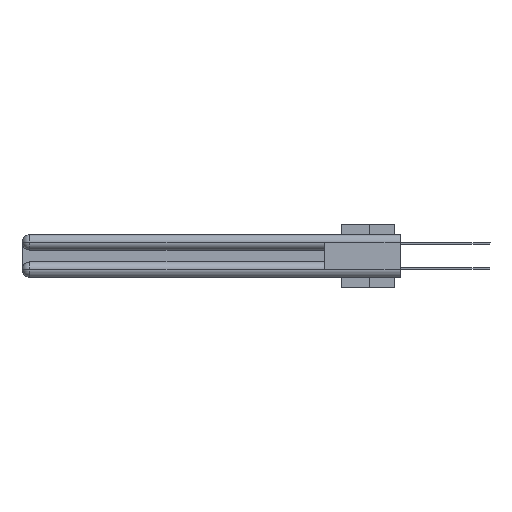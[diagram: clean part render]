
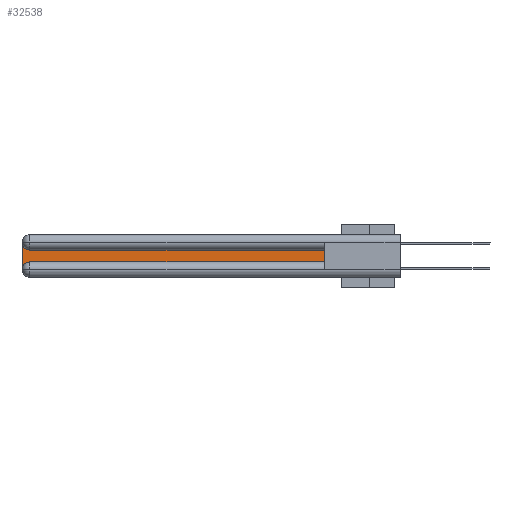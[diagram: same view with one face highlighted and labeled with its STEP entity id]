
A CAD part, left-side view. The second image highlights one B-rep face of the part: STEP entity #32538.
In plain terms, the highlighted planar face has unit normal (-1, 0, 0).
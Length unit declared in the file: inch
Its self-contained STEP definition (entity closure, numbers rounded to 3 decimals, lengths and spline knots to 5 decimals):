
#43 = AXIS2_PLACEMENT_3D ( 'NONE', #26752, #15834, #15995 ) ;
#588 = VECTOR ( 'NONE', #11236, 39.37008 ) ;
#1781 = DIRECTION ( 'NONE',  ( 1., 0., 0. ) ) ;
#1856 = VECTOR ( 'NONE', #23409, 39.37008 ) ;
#2509 = CARTESIAN_POINT ( 'NONE',  ( 0.075, 3., -0.2175 ) ) ;
#3250 = EDGE_CURVE ( 'NONE', #16935, #15985, #17031, .T. ) ;
#3287 = CIRCLE ( 'NONE', #22973, 0.06 ) ;
#3615 = ORIENTED_EDGE ( 'NONE', *, *, #17392, .T. ) ;
#4435 = CARTESIAN_POINT ( 'NONE',  ( 0.075, 3., -0.2775 ) ) ;
#5384 = FACE_OUTER_BOUND ( 'NONE', #6794, .T. ) ;
#5466 = VERTEX_POINT ( 'NONE', #32151 ) ;
#6429 = CARTESIAN_POINT ( 'NONE',  ( 0.075, 2.94, -0.0625 ) ) ;
#6794 = EDGE_LOOP ( 'NONE', ( #24310, #8093, #25225, #15275, #3615, #29367 ) ) ;
#6808 = VERTEX_POINT ( 'NONE', #4435 ) ;
#8093 = ORIENTED_EDGE ( 'NONE', *, *, #3250, .T. ) ;
#8192 = EDGE_CURVE ( 'NONE', #15985, #6808, #25975, .T. ) ;
#8545 = LINE ( 'NONE', #20891, #24804 ) ;
#8816 = LINE ( 'NONE', #26793, #588 ) ;
#10789 = DIRECTION ( 'NONE',  ( 0., -1., 0. ) ) ;
#11079 = CARTESIAN_POINT ( 'NONE',  ( 0.075, 0.6, -0.2175 ) ) ;
#11236 = DIRECTION ( 'NONE',  ( 0., 1., 0. ) ) ;
#12246 = DIRECTION ( 'NONE',  ( 0., 0., -1. ) ) ;
#14469 = DIRECTION ( 'NONE',  ( 0., 0., -1. ) ) ;
#14650 = DIRECTION ( 'NONE',  ( 1., 0., 0. ) ) ;
#15275 = ORIENTED_EDGE ( 'NONE', *, *, #26025, .T. ) ;
#15800 = CARTESIAN_POINT ( 'NONE',  ( 0.075, 2.94, -0.1225 ) ) ;
#15834 = DIRECTION ( 'NONE',  ( 1., 0., 0. ) ) ;
#15985 = VERTEX_POINT ( 'NONE', #25346 ) ;
#15995 = DIRECTION ( 'NONE',  ( 0., 0., -1. ) ) ;
#16935 = VERTEX_POINT ( 'NONE', #15800 ) ;
#17031 = CIRCLE ( 'NONE', #24674, 0.06 ) ;
#17318 = VECTOR ( 'NONE', #19879, 39.37008 ) ;
#17392 = EDGE_CURVE ( 'NONE', #20267, #17768, #8545, .T. ) ;
#17768 = VERTEX_POINT ( 'NONE', #11079 ) ;
#18297 = CARTESIAN_POINT ( 'NONE',  ( 0.075, 2.94, -0.2175 ) ) ;
#19879 = DIRECTION ( 'NONE',  ( 0., 0., 1. ) ) ;
#20267 = VERTEX_POINT ( 'NONE', #18297 ) ;
#20275 = EDGE_CURVE ( 'NONE', #17768, #5466, #33497, .T. ) ;
#20891 = CARTESIAN_POINT ( 'NONE',  ( 0.075, 0.6, -0.2175 ) ) ;
#22973 = AXIS2_PLACEMENT_3D ( 'NONE', #25266, #1781, #12246 ) ;
#23409 = DIRECTION ( 'NONE',  ( 0., 0., -1. ) ) ;
#24310 = ORIENTED_EDGE ( 'NONE', *, *, #32031, .T. ) ;
#24674 = AXIS2_PLACEMENT_3D ( 'NONE', #6429, #14650, #14469 ) ;
#24804 = VECTOR ( 'NONE', #10789, 39.37008 ) ;
#25225 = ORIENTED_EDGE ( 'NONE', *, *, #8192, .T. ) ;
#25266 = CARTESIAN_POINT ( 'NONE',  ( 0.075, 2.94, -0.2775 ) ) ;
#25346 = CARTESIAN_POINT ( 'NONE',  ( 0.075, 3., -0.0625 ) ) ;
#25975 = LINE ( 'NONE', #2509, #1856 ) ;
#26025 = EDGE_CURVE ( 'NONE', #6808, #20267, #3287, .T. ) ;
#26752 = CARTESIAN_POINT ( 'NONE',  ( 0.075, 3., -0.1225 ) ) ;
#26793 = CARTESIAN_POINT ( 'NONE',  ( 0.075, 0.6, -0.1225 ) ) ;
#28716 = CARTESIAN_POINT ( 'NONE',  ( 0.075, 0.6, -0.2175 ) ) ;
#29145 = PLANE ( 'NONE',  #43 ) ;
#29367 = ORIENTED_EDGE ( 'NONE', *, *, #20275, .T. ) ;
#32031 = EDGE_CURVE ( 'NONE', #5466, #16935, #8816, .T. ) ;
#32151 = CARTESIAN_POINT ( 'NONE',  ( 0.075, 0.6, -0.1225 ) ) ;
#32538 = ADVANCED_FACE ( 'NONE', ( #5384 ), #29145, .F. ) ;
#33497 = LINE ( 'NONE', #28716, #17318 ) ;
